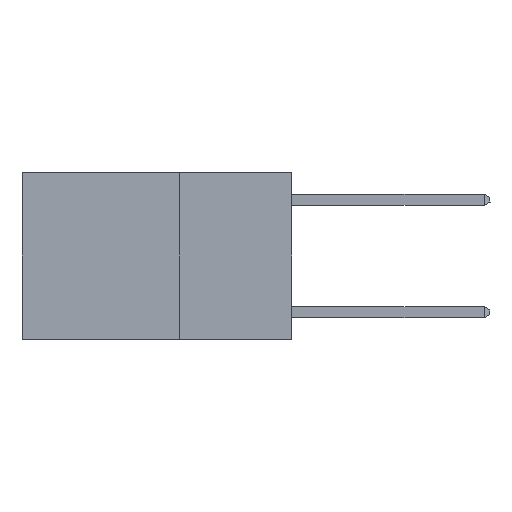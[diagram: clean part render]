
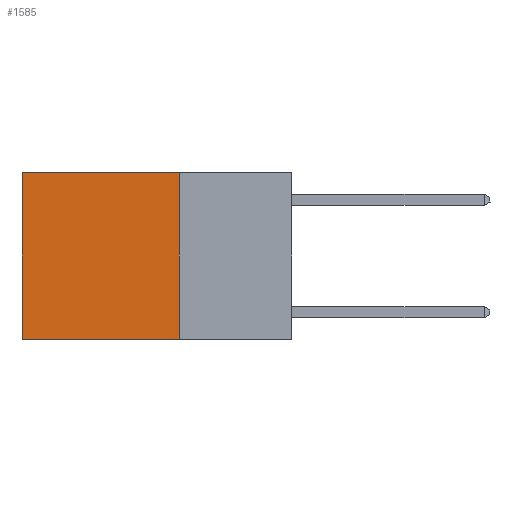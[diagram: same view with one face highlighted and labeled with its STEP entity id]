
A CAD part, left-side view. The second image highlights one B-rep face of the part: STEP entity #1585.
In plain terms, the highlighted planar face has unit normal (-1, 0, 0).
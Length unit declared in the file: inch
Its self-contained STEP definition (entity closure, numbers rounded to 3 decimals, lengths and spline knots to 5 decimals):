
#840 = DIRECTION ( 'NONE',  ( 0., 1., 0. ) ) ;
#1133 = VERTEX_POINT ( 'NONE', #6545 ) ;
#1395 = VECTOR ( 'NONE', #10013, 39.37008 ) ;
#1403 = CARTESIAN_POINT ( 'NONE',  ( 0.2625, 0.25, -0.37 ) ) ;
#1585 = ADVANCED_FACE ( 'NONE', ( #17653 ), #17393, .F. ) ;
#1618 = EDGE_CURVE ( 'NONE', #1133, #16441, #11312, .T. ) ;
#3758 = ORIENTED_EDGE ( 'NONE', *, *, #6011, .T. ) ;
#3795 = DIRECTION ( 'NONE',  ( 1., 0., 0. ) ) ;
#4044 = ORIENTED_EDGE ( 'NONE', *, *, #11885, .T. ) ;
#4542 = ORIENTED_EDGE ( 'NONE', *, *, #8675, .F. ) ;
#4546 = DIRECTION ( 'NONE',  ( 0., 0., -1. ) ) ;
#5056 = CARTESIAN_POINT ( 'NONE',  ( 0.2625, 0.6, 0. ) ) ;
#6011 = EDGE_CURVE ( 'NONE', #6687, #16441, #6173, .T. ) ;
#6173 = LINE ( 'NONE', #11345, #1395 ) ;
#6545 = CARTESIAN_POINT ( 'NONE',  ( 0.2625, 0.25, -0.37 ) ) ;
#6687 = VERTEX_POINT ( 'NONE', #5056 ) ;
#7119 = DIRECTION ( 'NONE',  ( 0., 1., 0. ) ) ;
#7867 = VECTOR ( 'NONE', #4546, 39.37008 ) ;
#7929 = DIRECTION ( 'NONE',  ( 0., 0., -1. ) ) ;
#8263 = ORIENTED_EDGE ( 'NONE', *, *, #1618, .F. ) ;
#8675 = EDGE_CURVE ( 'NONE', #12985, #1133, #16796, .T. ) ;
#8678 = AXIS2_PLACEMENT_3D ( 'NONE', #16076, #3795, #7929 ) ;
#10013 = DIRECTION ( 'NONE',  ( 0., 0., -1. ) ) ;
#10412 = LINE ( 'NONE', #14523, #11383 ) ;
#10902 = CARTESIAN_POINT ( 'NONE',  ( 0.2625, 0.25, 0. ) ) ;
#11009 = CARTESIAN_POINT ( 'NONE',  ( 0.2625, 0.25, 0. ) ) ;
#11312 = LINE ( 'NONE', #1403, #16107 ) ;
#11345 = CARTESIAN_POINT ( 'NONE',  ( 0.2625, 0.6, 0. ) ) ;
#11383 = VECTOR ( 'NONE', #840, 39.37008 ) ;
#11885 = EDGE_CURVE ( 'NONE', #12985, #6687, #10412, .T. ) ;
#12985 = VERTEX_POINT ( 'NONE', #10902 ) ;
#14465 = CARTESIAN_POINT ( 'NONE',  ( 0.2625, 0.6, -0.37 ) ) ;
#14523 = CARTESIAN_POINT ( 'NONE',  ( 0.2625, 0.25, 0. ) ) ;
#16076 = CARTESIAN_POINT ( 'NONE',  ( 0.2625, 0.25, 0. ) ) ;
#16107 = VECTOR ( 'NONE', #7119, 39.37008 ) ;
#16441 = VERTEX_POINT ( 'NONE', #14465 ) ;
#16796 = LINE ( 'NONE', #11009, #7867 ) ;
#17393 = PLANE ( 'NONE',  #8678 ) ;
#17502 = EDGE_LOOP ( 'NONE', ( #3758, #8263, #4542, #4044 ) ) ;
#17653 = FACE_OUTER_BOUND ( 'NONE', #17502, .T. ) ;
